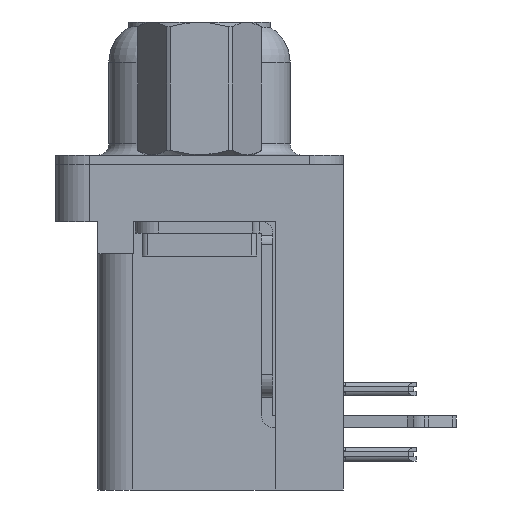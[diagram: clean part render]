
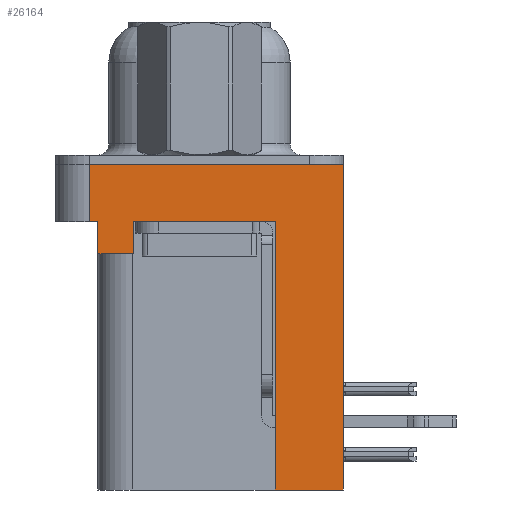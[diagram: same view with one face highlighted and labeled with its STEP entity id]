
A CAD part, left-side view. The second image highlights one B-rep face of the part: STEP entity #26164.
In plain terms, the highlighted planar face has unit normal (-1, 0, 0).
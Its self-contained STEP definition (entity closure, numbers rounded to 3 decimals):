
#1762 = FACE_OUTER_BOUND ( 'NONE', #7610, .T. ) ;
#1964 = VERTEX_POINT ( 'NONE', #19424 ) ;
#2433 = CARTESIAN_POINT ( 'NONE',  ( -3., -3.295, -14.2 ) ) ;
#2803 = DIRECTION ( 'NONE',  ( 0., 0., 1. ) ) ;
#3918 = EDGE_CURVE ( 'NONE', #35858, #9525, #31142, .T. ) ;
#4428 = CARTESIAN_POINT ( 'NONE',  ( -3., 4.775, -2.5 ) ) ;
#4522 = ORIENTED_EDGE ( 'NONE', *, *, #5605, .F. ) ;
#4642 = CARTESIAN_POINT ( 'NONE',  ( -3., -3.295, -2.5 ) ) ;
#4857 = DIRECTION ( 'NONE',  ( 0., -1., 0. ) ) ;
#5156 = CARTESIAN_POINT ( 'NONE',  ( -3., 4.775, -2.5 ) ) ;
#5605 = EDGE_CURVE ( 'NONE', #1964, #8454, #30390, .T. ) ;
#5945 = DIRECTION ( 'NONE',  ( 0., 0., 1. ) ) ;
#6041 = CARTESIAN_POINT ( 'NONE',  ( -3., -6.275, -2.5 ) ) ;
#6540 = ORIENTED_EDGE ( 'NONE', *, *, #29377, .F. ) ;
#6576 = ORIENTED_EDGE ( 'NONE', *, *, #3918, .T. ) ;
#7060 = CARTESIAN_POINT ( 'NONE',  ( -3., 2.895, -2.5 ) ) ;
#7099 = EDGE_CURVE ( 'NONE', #19655, #8706, #14423, .T. ) ;
#7610 = EDGE_LOOP ( 'NONE', ( #20389, #29438, #17035, #4522, #34629, #13792, #29651, #6540, #11514, #6576 ) ) ;
#8454 = VERTEX_POINT ( 'NONE', #24249 ) ;
#8697 = DIRECTION ( 'NONE',  ( 0., 1., 0. ) ) ;
#8706 = VERTEX_POINT ( 'NONE', #7060 ) ;
#9358 = PLANE ( 'NONE',  #11928 ) ;
#9525 = VERTEX_POINT ( 'NONE', #10028 ) ;
#9911 = CARTESIAN_POINT ( 'NONE',  ( -3., -6.275, -2.5 ) ) ;
#10028 = CARTESIAN_POINT ( 'NONE',  ( -3., -6.275, 0. ) ) ;
#10339 = DIRECTION ( 'NONE',  ( 0., 0., 1. ) ) ;
#10919 = VERTEX_POINT ( 'NONE', #35738 ) ;
#11514 = ORIENTED_EDGE ( 'NONE', *, *, #17176, .F. ) ;
#11517 = VERTEX_POINT ( 'NONE', #16873 ) ;
#11928 = AXIS2_PLACEMENT_3D ( 'NONE', #9911, #34789, #18009 ) ;
#12851 = VECTOR ( 'NONE', #15065, 1000. ) ;
#12961 = CARTESIAN_POINT ( 'NONE',  ( -3., 2.895, -3.9 ) ) ;
#13066 = EDGE_CURVE ( 'NONE', #22567, #8454, #16818, .T. ) ;
#13792 = ORIENTED_EDGE ( 'NONE', *, *, #7099, .T. ) ;
#14324 = VECTOR ( 'NONE', #5945, 1000. ) ;
#14423 = LINE ( 'NONE', #22547, #14324 ) ;
#14571 = LINE ( 'NONE', #33962, #16235 ) ;
#14617 = VERTEX_POINT ( 'NONE', #4642 ) ;
#14897 = VECTOR ( 'NONE', #10339, 1000. ) ;
#15065 = DIRECTION ( 'NONE',  ( 0., -1., 0. ) ) ;
#15527 = VECTOR ( 'NONE', #2803, 1000. ) ;
#15684 = EDGE_CURVE ( 'NONE', #19655, #1964, #31333, .T. ) ;
#16235 = VECTOR ( 'NONE', #8697, 1000. ) ;
#16818 = LINE ( 'NONE', #19216, #27927 ) ;
#16873 = CARTESIAN_POINT ( 'NONE',  ( -3., -3.295, -14.2 ) ) ;
#17035 = ORIENTED_EDGE ( 'NONE', *, *, #13066, .T. ) ;
#17123 = CARTESIAN_POINT ( 'NONE',  ( -3., -6.275, -2.5 ) ) ;
#17176 = EDGE_CURVE ( 'NONE', #35858, #11517, #14571, .T. ) ;
#18009 = DIRECTION ( 'NONE',  ( 0., 0., 1. ) ) ;
#19216 = CARTESIAN_POINT ( 'NONE',  ( -3., -6.275, -2.5 ) ) ;
#19424 = CARTESIAN_POINT ( 'NONE',  ( -3., 4.425, -3.9 ) ) ;
#19576 = LINE ( 'NONE', #2433, #15527 ) ;
#19655 = VERTEX_POINT ( 'NONE', #12961 ) ;
#19915 = CARTESIAN_POINT ( 'NONE',  ( -3., -6.275, 0. ) ) ;
#19974 = VECTOR ( 'NONE', #20257, 1000. ) ;
#20137 = EDGE_CURVE ( 'NONE', #10919, #9525, #33575, .T. ) ;
#20235 = LINE ( 'NONE', #6041, #12851 ) ;
#20257 = DIRECTION ( 'NONE',  ( 0., 0., 1. ) ) ;
#20389 = ORIENTED_EDGE ( 'NONE', *, *, #20137, .F. ) ;
#21566 = LINE ( 'NONE', #5156, #14897 ) ;
#21625 = EDGE_CURVE ( 'NONE', #8706, #14617, #20235, .T. ) ;
#22489 = CARTESIAN_POINT ( 'NONE',  ( -3., -6.275, -14.2 ) ) ;
#22494 = DIRECTION ( 'NONE',  ( 0., -1., 0. ) ) ;
#22547 = CARTESIAN_POINT ( 'NONE',  ( -3., 2.895, -3.9 ) ) ;
#22567 = VERTEX_POINT ( 'NONE', #4428 ) ;
#24249 = CARTESIAN_POINT ( 'NONE',  ( -3., 4.425, -2.5 ) ) ;
#25636 = DIRECTION ( 'NONE',  ( 0., 1., 0. ) ) ;
#26164 = ADVANCED_FACE ( 'NONE', ( #1762 ), #9358, .T. ) ;
#27344 = VECTOR ( 'NONE', #25636, 1000. ) ;
#27927 = VECTOR ( 'NONE', #4857, 1000. ) ;
#28698 = VECTOR ( 'NONE', #22494, 1000. ) ;
#28912 = EDGE_CURVE ( 'NONE', #22567, #10919, #21566, .T. ) ;
#29377 = EDGE_CURVE ( 'NONE', #11517, #14617, #19576, .T. ) ;
#29438 = ORIENTED_EDGE ( 'NONE', *, *, #28912, .F. ) ;
#29651 = ORIENTED_EDGE ( 'NONE', *, *, #21625, .T. ) ;
#30390 = LINE ( 'NONE', #33345, #33753 ) ;
#30566 = DIRECTION ( 'NONE',  ( 0., 0., 1. ) ) ;
#31142 = LINE ( 'NONE', #17123, #19974 ) ;
#31333 = LINE ( 'NONE', #34124, #27344 ) ;
#33345 = CARTESIAN_POINT ( 'NONE',  ( -3., 4.425, -3.9 ) ) ;
#33575 = LINE ( 'NONE', #19915, #28698 ) ;
#33753 = VECTOR ( 'NONE', #30566, 1000. ) ;
#33962 = CARTESIAN_POINT ( 'NONE',  ( -3., -3.295, -14.2 ) ) ;
#34124 = CARTESIAN_POINT ( 'NONE',  ( -3., 4.425, -3.9 ) ) ;
#34629 = ORIENTED_EDGE ( 'NONE', *, *, #15684, .F. ) ;
#34789 = DIRECTION ( 'NONE',  ( -1., 0., 0. ) ) ;
#35738 = CARTESIAN_POINT ( 'NONE',  ( -3., 4.775, 0. ) ) ;
#35858 = VERTEX_POINT ( 'NONE', #22489 ) ;
